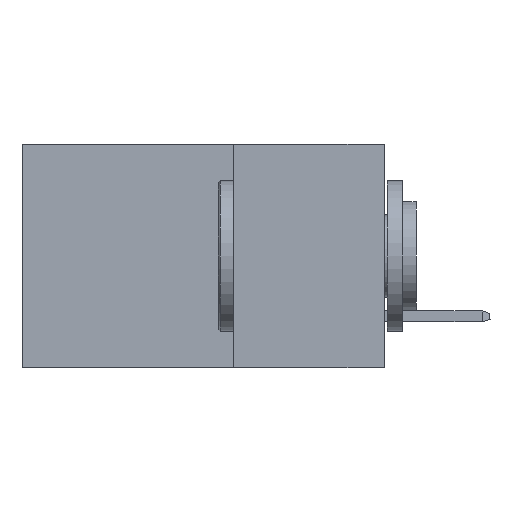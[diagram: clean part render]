
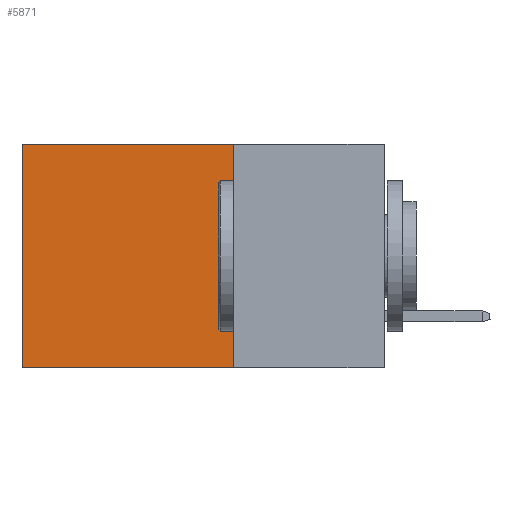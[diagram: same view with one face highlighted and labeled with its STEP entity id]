
A CAD part, left-side view. The second image highlights one B-rep face of the part: STEP entity #5871.
In plain terms, the highlighted planar face has unit normal (-1, 0, 0).
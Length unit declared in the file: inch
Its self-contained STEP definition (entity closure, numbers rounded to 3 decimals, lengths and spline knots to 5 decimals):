
#1340 = AXIS2_PLACEMENT_3D ( 'NONE', #18963, #1343, #27741 ) ;
#1343 = DIRECTION ( 'NONE',  ( 1., 0., 0. ) ) ;
#1416 = LINE ( 'NONE', #3259, #26312 ) ;
#1646 = EDGE_CURVE ( 'NONE', #14031, #9828, #18176, .T. ) ;
#2572 = FACE_OUTER_BOUND ( 'NONE', #8281, .T. ) ;
#3259 = CARTESIAN_POINT ( 'NONE',  ( 0.298, 0.6, 0. ) ) ;
#3460 = LINE ( 'NONE', #15971, #23261 ) ;
#3571 = ORIENTED_EDGE ( 'NONE', *, *, #1646, .T. ) ;
#5871 = ADVANCED_FACE ( 'NONE', ( #2572 ), #23176, .F. ) ;
#7759 = CARTESIAN_POINT ( 'NONE',  ( 0.298, 0.6, -0.37 ) ) ;
#8281 = EDGE_LOOP ( 'NONE', ( #26277, #17746, #21370, #3571 ) ) ;
#8764 = EDGE_CURVE ( 'NONE', #14031, #15869, #3460, .T. ) ;
#8932 = EDGE_CURVE ( 'NONE', #9828, #23933, #1416, .T. ) ;
#9828 = VERTEX_POINT ( 'NONE', #12530 ) ;
#12231 = CARTESIAN_POINT ( 'NONE',  ( 0.298, 0.25, -0.37 ) ) ;
#12530 = CARTESIAN_POINT ( 'NONE',  ( 0.298, 0.6, 0. ) ) ;
#13439 = VECTOR ( 'NONE', #21899, 39.37008 ) ;
#14031 = VERTEX_POINT ( 'NONE', #18203 ) ;
#15869 = VERTEX_POINT ( 'NONE', #12231 ) ;
#15971 = CARTESIAN_POINT ( 'NONE',  ( 0.298, 0.25, 0. ) ) ;
#16417 = LINE ( 'NONE', #27889, #19148 ) ;
#17746 = ORIENTED_EDGE ( 'NONE', *, *, #26297, .F. ) ;
#18176 = LINE ( 'NONE', #19526, #13439 ) ;
#18203 = CARTESIAN_POINT ( 'NONE',  ( 0.298, 0.25, 0. ) ) ;
#18963 = CARTESIAN_POINT ( 'NONE',  ( 0.298, 0.25, 0. ) ) ;
#19148 = VECTOR ( 'NONE', #23524, 39.37008 ) ;
#19526 = CARTESIAN_POINT ( 'NONE',  ( 0.298, 0.25, 0. ) ) ;
#20414 = DIRECTION ( 'NONE',  ( 0., 0., -1. ) ) ;
#21370 = ORIENTED_EDGE ( 'NONE', *, *, #8764, .F. ) ;
#21899 = DIRECTION ( 'NONE',  ( 0., 1., 0. ) ) ;
#23176 = PLANE ( 'NONE',  #1340 ) ;
#23261 = VECTOR ( 'NONE', #20414, 39.37008 ) ;
#23524 = DIRECTION ( 'NONE',  ( 0., 1., 0. ) ) ;
#23933 = VERTEX_POINT ( 'NONE', #7759 ) ;
#24703 = DIRECTION ( 'NONE',  ( 0., 0., -1. ) ) ;
#26277 = ORIENTED_EDGE ( 'NONE', *, *, #8932, .T. ) ;
#26297 = EDGE_CURVE ( 'NONE', #15869, #23933, #16417, .T. ) ;
#26312 = VECTOR ( 'NONE', #24703, 39.37008 ) ;
#27741 = DIRECTION ( 'NONE',  ( 0., 0., -1. ) ) ;
#27889 = CARTESIAN_POINT ( 'NONE',  ( 0.298, 0.25, -0.37 ) ) ;
